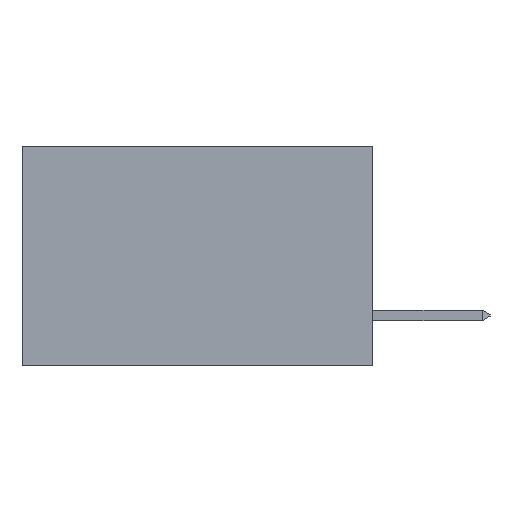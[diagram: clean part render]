
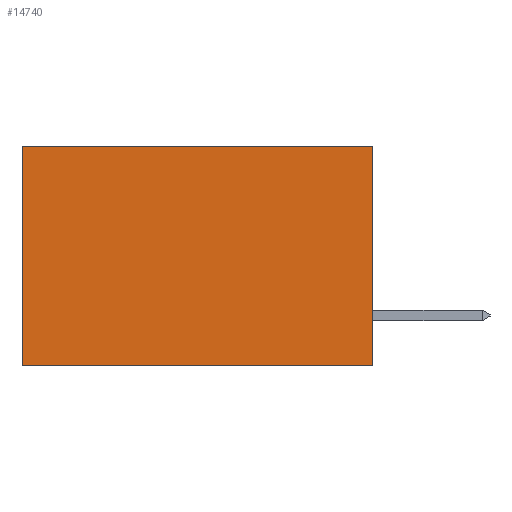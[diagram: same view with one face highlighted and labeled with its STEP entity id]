
A CAD part, left-side view. The second image highlights one B-rep face of the part: STEP entity #14740.
In plain terms, the highlighted planar face has unit normal (-1, 0, 0).
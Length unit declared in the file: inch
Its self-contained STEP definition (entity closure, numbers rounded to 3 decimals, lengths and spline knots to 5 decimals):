
#1174 = PLANE ( 'NONE',  #19401 ) ;
#1693 = CARTESIAN_POINT ( 'NONE',  ( 0.277, 0., -0.37 ) ) ;
#2472 = LINE ( 'NONE', #24303, #20230 ) ;
#2535 = VECTOR ( 'NONE', #21264, 39.37008 ) ;
#2737 = CARTESIAN_POINT ( 'NONE',  ( 0.277, 0., -0.37 ) ) ;
#4527 = EDGE_LOOP ( 'NONE', ( #6134, #13623, #21894, #13920 ) ) ;
#4989 = LINE ( 'NONE', #17888, #22711 ) ;
#5821 = DIRECTION ( 'NONE',  ( 1., 0., 0. ) ) ;
#6134 = ORIENTED_EDGE ( 'NONE', *, *, #14761, .T. ) ;
#8665 = DIRECTION ( 'NONE',  ( 0., 1., 0. ) ) ;
#9486 = VERTEX_POINT ( 'NONE', #15642 ) ;
#10262 = VERTEX_POINT ( 'NONE', #23126 ) ;
#12791 = DIRECTION ( 'NONE',  ( 0., 0., -1. ) ) ;
#13623 = ORIENTED_EDGE ( 'NONE', *, *, #23177, .F. ) ;
#13902 = EDGE_CURVE ( 'NONE', #9486, #15517, #22423, .T. ) ;
#13920 = ORIENTED_EDGE ( 'NONE', *, *, #14864, .T. ) ;
#14740 = ADVANCED_FACE ( 'NONE', ( #26958 ), #1174, .F. ) ;
#14761 = EDGE_CURVE ( 'NONE', #28667, #10262, #2472, .T. ) ;
#14864 = EDGE_CURVE ( 'NONE', #9486, #28667, #4989, .T. ) ;
#15056 = VECTOR ( 'NONE', #8665, 39.37008 ) ;
#15517 = VERTEX_POINT ( 'NONE', #20282 ) ;
#15642 = CARTESIAN_POINT ( 'NONE',  ( 0.277, 0., 0. ) ) ;
#15776 = LINE ( 'NONE', #1693, #15056 ) ;
#17888 = CARTESIAN_POINT ( 'NONE',  ( 0.277, 0., 0. ) ) ;
#19401 = AXIS2_PLACEMENT_3D ( 'NONE', #19702, #5821, #22004 ) ;
#19702 = CARTESIAN_POINT ( 'NONE',  ( 0.277, 0., -0.37 ) ) ;
#20202 = DIRECTION ( 'NONE',  ( 0., 1., 0. ) ) ;
#20230 = VECTOR ( 'NONE', #12791, 39.37008 ) ;
#20282 = CARTESIAN_POINT ( 'NONE',  ( 0.277, 0., -0.37 ) ) ;
#21264 = DIRECTION ( 'NONE',  ( 0., 0., -1. ) ) ;
#21894 = ORIENTED_EDGE ( 'NONE', *, *, #13902, .F. ) ;
#22004 = DIRECTION ( 'NONE',  ( 0., 0., -1. ) ) ;
#22423 = LINE ( 'NONE', #2737, #2535 ) ;
#22711 = VECTOR ( 'NONE', #20202, 39.37008 ) ;
#22769 = CARTESIAN_POINT ( 'NONE',  ( 0.277, 0.59, 0. ) ) ;
#23126 = CARTESIAN_POINT ( 'NONE',  ( 0.277, 0.59, -0.37 ) ) ;
#23177 = EDGE_CURVE ( 'NONE', #15517, #10262, #15776, .T. ) ;
#24303 = CARTESIAN_POINT ( 'NONE',  ( 0.277, 0.59, -0.37 ) ) ;
#26958 = FACE_OUTER_BOUND ( 'NONE', #4527, .T. ) ;
#28667 = VERTEX_POINT ( 'NONE', #22769 ) ;
